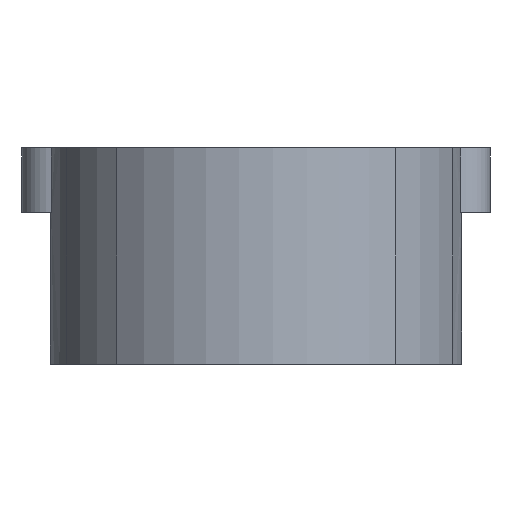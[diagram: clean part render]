
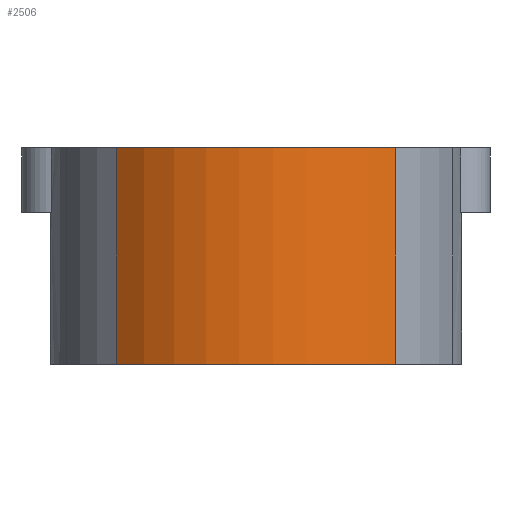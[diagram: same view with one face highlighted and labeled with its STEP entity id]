
A CAD part, left-side view. The second image highlights one B-rep face of the part: STEP entity #2506.
In plain terms, the highlighted cylindrical face has radius 31.9 mm (diameter 63.8 mm), a partial arc.
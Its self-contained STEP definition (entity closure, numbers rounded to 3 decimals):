
#104 = PLANE('',#105);
#105 = AXIS2_PLACEMENT_3D('',#106,#107,#108);
#106 = CARTESIAN_POINT('',(52.832,57.019,36.889));
#107 = DIRECTION('',(0.,0.,1.));
#108 = DIRECTION('',(0.,-1.,0.));
#804 = VERTEX_POINT('',#805);
#805 = CARTESIAN_POINT('',(-24.584,40.,36.889));
#820 = CYLINDRICAL_SURFACE('',#821,31.9);
#821 = AXIS2_PLACEMENT_3D('',#822,#823,#824);
#822 = CARTESIAN_POINT('',(-0.988,18.534,36.957));
#823 = DIRECTION('',(0.,0.,1.));
#824 = DIRECTION('',(1.,0.,0.));
#832 = EDGE_CURVE('',#804,#833,#835,.T.);
#833 = VERTEX_POINT('',#834);
#834 = CARTESIAN_POINT('',(-24.523,-3.,36.889));
#835 = SURFACE_CURVE('',#836,(#841,#848),.PCURVE_S1.);
#836 = CIRCLE('',#837,31.9);
#837 = AXIS2_PLACEMENT_3D('',#838,#839,#840);
#838 = CARTESIAN_POINT('',(-0.988,18.534,36.889));
#839 = DIRECTION('',(0.,0.,1.));
#840 = DIRECTION('',(1.,0.,0.));
#841 = PCURVE('',#104,#842);
#842 = DEFINITIONAL_REPRESENTATION('',(#843),#847);
#843 = CIRCLE('',#844,31.9);
#844 = AXIS2_PLACEMENT_2D('',#845,#846);
#845 = CARTESIAN_POINT('',(38.485,-53.82));
#846 = DIRECTION('',(0.,1.));
#847 = ( GEOMETRIC_REPRESENTATION_CONTEXT(2) 
PARAMETRIC_REPRESENTATION_CONTEXT() REPRESENTATION_CONTEXT('2D SPACE',''
  ) );
#848 = PCURVE('',#849,#854);
#849 = CYLINDRICAL_SURFACE('',#850,31.9);
#850 = AXIS2_PLACEMENT_3D('',#851,#852,#853);
#851 = CARTESIAN_POINT('',(-0.988,18.534,36.957));
#852 = DIRECTION('',(0.,0.,1.));
#853 = DIRECTION('',(1.,0.,0.));
#854 = DEFINITIONAL_REPRESENTATION('',(#855),#859);
#855 = LINE('',#856,#857);
#856 = CARTESIAN_POINT('',(0.,-0.068));
#857 = VECTOR('',#858,1.);
#858 = DIRECTION('',(1.,0.));
#859 = ( GEOMETRIC_REPRESENTATION_CONTEXT(2) 
PARAMETRIC_REPRESENTATION_CONTEXT() REPRESENTATION_CONTEXT('2D SPACE',''
  ) );
#882 = CYLINDRICAL_SURFACE('',#883,31.9);
#883 = AXIS2_PLACEMENT_3D('',#884,#885,#886);
#884 = CARTESIAN_POINT('',(-0.988,18.534,3.611));
#885 = DIRECTION('',(0.,0.,-1.));
#886 = DIRECTION('',(1.,0.,0.));
#2458 = VERTEX_POINT('',#2459);
#2459 = CARTESIAN_POINT('',(-24.523,-3.,3.611));
#2485 = EDGE_CURVE('',#833,#2458,#2486,.T.);
#2486 = SURFACE_CURVE('',#2487,(#2491,#2497),.PCURVE_S1.);
#2487 = LINE('',#2488,#2489);
#2488 = CARTESIAN_POINT('',(-24.523,-3.,3.611));
#2489 = VECTOR('',#2490,1.);
#2490 = DIRECTION('',(0.,0.,-1.));
#2491 = PCURVE('',#882,#2492);
#2492 = DEFINITIONAL_REPRESENTATION('',(#2493),#2496);
#2493 = B_SPLINE_CURVE_WITH_KNOTS('',1,(#2494,#2495),.UNSPECIFIED.,.F.,
  .F.,(2,2),(-33.34,0.),.PIECEWISE_BEZIER_KNOTS.);
#2494 = CARTESIAN_POINT('',(-3.883,-33.34));
#2495 = CARTESIAN_POINT('',(-3.883,0.));
#2496 = ( GEOMETRIC_REPRESENTATION_CONTEXT(2) 
PARAMETRIC_REPRESENTATION_CONTEXT() REPRESENTATION_CONTEXT('2D SPACE',''
  ) );
#2497 = PCURVE('',#849,#2498);
#2498 = DEFINITIONAL_REPRESENTATION('',(#2499),#2503);
#2499 = LINE('',#2500,#2501);
#2500 = CARTESIAN_POINT('',(3.883,-33.346));
#2501 = VECTOR('',#2502,1.);
#2502 = DIRECTION('',(0.,-1.));
#2503 = ( GEOMETRIC_REPRESENTATION_CONTEXT(2) 
PARAMETRIC_REPRESENTATION_CONTEXT() REPRESENTATION_CONTEXT('2D SPACE',''
  ) );
#2506 = ADVANCED_FACE('',(#2507),#849,.T.);
#2507 = FACE_BOUND('',#2508,.T.);
#2508 = EDGE_LOOP('',(#2509,#2510,#2533,#2564));
#2509 = ORIENTED_EDGE('',*,*,#832,.F.);
#2510 = ORIENTED_EDGE('',*,*,#2511,.T.);
#2511 = EDGE_CURVE('',#804,#2512,#2514,.T.);
#2512 = VERTEX_POINT('',#2513);
#2513 = CARTESIAN_POINT('',(-24.584,40.,3.611));
#2514 = SURFACE_CURVE('',#2515,(#2519,#2526),.PCURVE_S1.);
#2515 = LINE('',#2516,#2517);
#2516 = CARTESIAN_POINT('',(-24.584,40.,3.611));
#2517 = VECTOR('',#2518,1.);
#2518 = DIRECTION('',(0.,0.,-1.));
#2519 = PCURVE('',#849,#2520);
#2520 = DEFINITIONAL_REPRESENTATION('',(#2521),#2525);
#2521 = LINE('',#2522,#2523);
#2522 = CARTESIAN_POINT('',(2.403,-33.346));
#2523 = VECTOR('',#2524,1.);
#2524 = DIRECTION('',(0.,-1.));
#2525 = ( GEOMETRIC_REPRESENTATION_CONTEXT(2) 
PARAMETRIC_REPRESENTATION_CONTEXT() REPRESENTATION_CONTEXT('2D SPACE',''
  ) );
#2526 = PCURVE('',#820,#2527);
#2527 = DEFINITIONAL_REPRESENTATION('',(#2528),#2532);
#2528 = LINE('',#2529,#2530);
#2529 = CARTESIAN_POINT('',(2.403,-33.346));
#2530 = VECTOR('',#2531,1.);
#2531 = DIRECTION('',(0.,-1.));
#2532 = ( GEOMETRIC_REPRESENTATION_CONTEXT(2) 
PARAMETRIC_REPRESENTATION_CONTEXT() REPRESENTATION_CONTEXT('2D SPACE',''
  ) );
#2533 = ORIENTED_EDGE('',*,*,#2534,.T.);
#2534 = EDGE_CURVE('',#2512,#2458,#2535,.T.);
#2535 = SURFACE_CURVE('',#2536,(#2541,#2548),.PCURVE_S1.);
#2536 = CIRCLE('',#2537,31.9);
#2537 = AXIS2_PLACEMENT_3D('',#2538,#2539,#2540);
#2538 = CARTESIAN_POINT('',(-0.988,18.534,3.611));
#2539 = DIRECTION('',(0.,0.,1.));
#2540 = DIRECTION('',(1.,0.,0.));
#2541 = PCURVE('',#849,#2542);
#2542 = DEFINITIONAL_REPRESENTATION('',(#2543),#2547);
#2543 = LINE('',#2544,#2545);
#2544 = CARTESIAN_POINT('',(0.,-33.346));
#2545 = VECTOR('',#2546,1.);
#2546 = DIRECTION('',(1.,0.));
#2547 = ( GEOMETRIC_REPRESENTATION_CONTEXT(2) 
PARAMETRIC_REPRESENTATION_CONTEXT() REPRESENTATION_CONTEXT('2D SPACE',''
  ) );
#2548 = PCURVE('',#2549,#2554);
#2549 = PLANE('',#2550);
#2550 = AXIS2_PLACEMENT_3D('',#2551,#2552,#2553);
#2551 = CARTESIAN_POINT('',(-41.749,-3.,3.611));
#2552 = DIRECTION('',(0.,0.,-1.));
#2553 = DIRECTION('',(1.,0.,0.));
#2554 = DEFINITIONAL_REPRESENTATION('',(#2555),#2563);
#2555 = ( BOUNDED_CURVE() B_SPLINE_CURVE(2,(#2556,#2557,#2558,#2559,
#2560,#2561,#2562),.UNSPECIFIED.,.F.,.F.) B_SPLINE_CURVE_WITH_KNOTS((1,2
    ,2,2,2,1),(-2.094,0.,2.094,4.189,
6.283,8.378),.UNSPECIFIED.) CURVE() 
GEOMETRIC_REPRESENTATION_ITEM() RATIONAL_B_SPLINE_CURVE((1.,0.5,1.,0.5,
1.,0.5,1.)) REPRESENTATION_ITEM('') );
#2556 = CARTESIAN_POINT('',(72.661,-21.534));
#2557 = CARTESIAN_POINT('',(72.661,-76.786));
#2558 = CARTESIAN_POINT('',(24.811,-49.16));
#2559 = CARTESIAN_POINT('',(-23.039,-21.534));
#2560 = CARTESIAN_POINT('',(24.811,6.093));
#2561 = CARTESIAN_POINT('',(72.661,33.719));
#2562 = CARTESIAN_POINT('',(72.661,-21.534));
#2563 = ( GEOMETRIC_REPRESENTATION_CONTEXT(2) 
PARAMETRIC_REPRESENTATION_CONTEXT() REPRESENTATION_CONTEXT('2D SPACE',''
  ) );
#2564 = ORIENTED_EDGE('',*,*,#2485,.F.);
